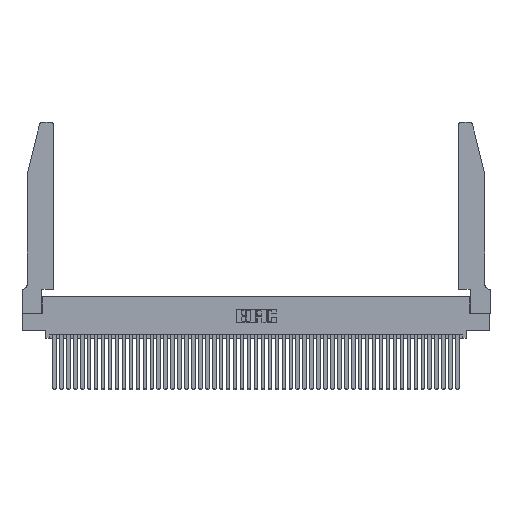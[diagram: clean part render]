
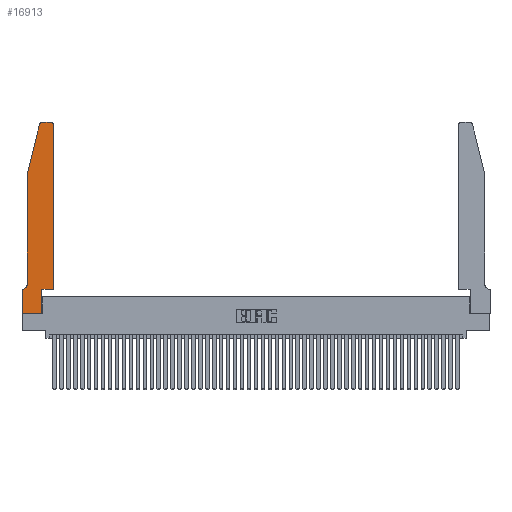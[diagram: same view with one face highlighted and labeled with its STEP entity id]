
A CAD part, top view. The second image highlights one B-rep face of the part: STEP entity #16913.
In plain terms, the highlighted planar face has unit normal (0, 0, 1).
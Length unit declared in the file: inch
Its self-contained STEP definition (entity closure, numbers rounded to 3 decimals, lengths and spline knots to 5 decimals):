
#142 = CARTESIAN_POINT ( 'NONE',  ( 0.25487, 2.72718, 0.37 ) ) ;
#521 = DIRECTION ( 'NONE',  ( 0., 1., 0. ) ) ;
#525 = LINE ( 'NONE', #27015, #20551 ) ;
#769 = VERTEX_POINT ( 'NONE', #40874 ) ;
#1063 = VECTOR ( 'NONE', #29589, 39.37008 ) ;
#1357 = ORIENTED_EDGE ( 'NONE', *, *, #36093, .T. ) ;
#1741 = EDGE_CURVE ( 'NONE', #16546, #47870, #20630, .T. ) ;
#1977 = DIRECTION ( 'NONE',  ( 0., 1., 0. ) ) ;
#2802 = EDGE_CURVE ( 'NONE', #31065, #769, #28888, .T. ) ;
#2891 = ORIENTED_EDGE ( 'NONE', *, *, #9325, .T. ) ;
#2956 = EDGE_CURVE ( 'NONE', #36001, #34604, #525, .T. ) ;
#3140 = VECTOR ( 'NONE', #14003, 39.37008 ) ;
#3671 = EDGE_CURVE ( 'NONE', #769, #18254, #16994, .T. ) ;
#3911 = EDGE_CURVE ( 'NONE', #32837, #31065, #13444, .T. ) ;
#4272 = DIRECTION ( 'NONE',  ( 1., 0., 0. ) ) ;
#4958 = DIRECTION ( 'NONE',  ( 1., 0., 0. ) ) ;
#6126 = DIRECTION ( 'NONE',  ( 0., 0., 1. ) ) ;
#7784 = VERTEX_POINT ( 'NONE', #32909 ) ;
#7906 = VECTOR ( 'NONE', #19432, 39.37008 ) ;
#8168 = CARTESIAN_POINT ( 'NONE',  ( 0.0755, 2., 0.37 ) ) ;
#8601 = EDGE_LOOP ( 'NONE', ( #1357, #22164, #12713, #36730, #45489, #14178, #24585, #2891, #27824, #33844, #46316, #10933 ) ) ;
#9325 = EDGE_CURVE ( 'NONE', #38260, #18668, #43754, .T. ) ;
#9332 = CARTESIAN_POINT ( 'NONE',  ( 0., 0.35, 0.37 ) ) ;
#9610 = CARTESIAN_POINT ( 'NONE',  ( 0., 0.35, 0.37 ) ) ;
#10315 = VERTEX_POINT ( 'NONE', #19049 ) ;
#10933 = ORIENTED_EDGE ( 'NONE', *, *, #25703, .T. ) ;
#12238 = VECTOR ( 'NONE', #23184, 39.37008 ) ;
#12713 = ORIENTED_EDGE ( 'NONE', *, *, #17390, .T. ) ;
#13444 = LINE ( 'NONE', #22144, #1063 ) ;
#14003 = DIRECTION ( 'NONE',  ( -1., 0., 0. ) ) ;
#14178 = ORIENTED_EDGE ( 'NONE', *, *, #3671, .T. ) ;
#14229 = CARTESIAN_POINT ( 'NONE',  ( 0.0755, 0.35, 0.37 ) ) ;
#14549 = CARTESIAN_POINT ( 'NONE',  ( 0.4205, 2.72, 0.37 ) ) ;
#14589 = VECTOR ( 'NONE', #1977, 39.37008 ) ;
#15662 = CARTESIAN_POINT ( 'NONE',  ( 0.0755, 2., 0.37 ) ) ;
#16546 = VERTEX_POINT ( 'NONE', #43193 ) ;
#16913 = ADVANCED_FACE ( 'NONE', ( #31694 ), #40052, .T. ) ;
#16994 = LINE ( 'NONE', #14229, #44630 ) ;
#17390 = EDGE_CURVE ( 'NONE', #47870, #32837, #26943, .T. ) ;
#17442 = EDGE_CURVE ( 'NONE', #18668, #10315, #37560, .T. ) ;
#17662 = DIRECTION ( 'NONE',  ( 1., 0., 0. ) ) ;
#17706 = DIRECTION ( 'NONE',  ( -1., 0., 0. ) ) ;
#18254 = VERTEX_POINT ( 'NONE', #9332 ) ;
#18338 = DIRECTION ( 'NONE',  ( 0., 0., -1. ) ) ;
#18668 = VERTEX_POINT ( 'NONE', #41861 ) ;
#19049 = CARTESIAN_POINT ( 'NONE',  ( 0.2865, 0.35, 0.37 ) ) ;
#19432 = DIRECTION ( 'NONE',  ( 0., -1., 0. ) ) ;
#19603 = CARTESIAN_POINT ( 'NONE',  ( 0., 0., 0.37 ) ) ;
#20551 = VECTOR ( 'NONE', #521, 39.37008 ) ;
#20630 = CIRCLE ( 'NONE', #36042, 0.03 ) ;
#22144 = CARTESIAN_POINT ( 'NONE',  ( 0.0755, 2., 0.37 ) ) ;
#22164 = ORIENTED_EDGE ( 'NONE', *, *, #1741, .T. ) ;
#22322 = CARTESIAN_POINT ( 'NONE',  ( 0., 0., 0.37 ) ) ;
#22633 = CARTESIAN_POINT ( 'NONE',  ( 0.4505, 2.72, 0.37 ) ) ;
#22659 = EDGE_CURVE ( 'NONE', #18254, #38260, #39142, .T. ) ;
#23184 = DIRECTION ( 'NONE',  ( -0.239, -0.971, 0. ) ) ;
#24585 = ORIENTED_EDGE ( 'NONE', *, *, #22659, .T. ) ;
#25005 = CARTESIAN_POINT ( 'NONE',  ( 0.4505, 0.35, 0.37 ) ) ;
#25560 = DIRECTION ( 'NONE',  ( 0., 0., 1. ) ) ;
#25703 = EDGE_CURVE ( 'NONE', #34604, #7784, #44085, .T. ) ;
#25897 = VECTOR ( 'NONE', #29331, 39.37008 ) ;
#26943 = LINE ( 'NONE', #15662, #12238 ) ;
#27015 = CARTESIAN_POINT ( 'NONE',  ( 0.4505, 0.35, 0.37 ) ) ;
#27170 = CARTESIAN_POINT ( 'NONE',  ( 0.284, 2.72, 0.37 ) ) ;
#27824 = ORIENTED_EDGE ( 'NONE', *, *, #17442, .T. ) ;
#28054 = AXIS2_PLACEMENT_3D ( 'NONE', #14549, #25560, #47782 ) ;
#28888 = CIRCLE ( 'NONE', #38283, 0.07 ) ;
#29331 = DIRECTION ( 'NONE',  ( 1., 0., 0. ) ) ;
#29589 = DIRECTION ( 'NONE',  ( 0., -1., 0. ) ) ;
#31065 = VERTEX_POINT ( 'NONE', #43310 ) ;
#31694 = FACE_OUTER_BOUND ( 'NONE', #8601, .T. ) ;
#32837 = VERTEX_POINT ( 'NONE', #8168 ) ;
#32909 = CARTESIAN_POINT ( 'NONE',  ( 0.4205, 2.75, 0.37 ) ) ;
#33058 = LINE ( 'NONE', #48221, #25897 ) ;
#33844 = ORIENTED_EDGE ( 'NONE', *, *, #42721, .T. ) ;
#34604 = VERTEX_POINT ( 'NONE', #22633 ) ;
#35227 = CARTESIAN_POINT ( 'NONE',  ( 0.2865, 0.35, 0.37 ) ) ;
#35390 = AXIS2_PLACEMENT_3D ( 'NONE', #9610, #6126, #17662 ) ;
#36001 = VERTEX_POINT ( 'NONE', #25005 ) ;
#36042 = AXIS2_PLACEMENT_3D ( 'NONE', #27170, #46253, #4958 ) ;
#36093 = EDGE_CURVE ( 'NONE', #7784, #16546, #37879, .T. ) ;
#36730 = ORIENTED_EDGE ( 'NONE', *, *, #3911, .T. ) ;
#37560 = LINE ( 'NONE', #35227, #14589 ) ;
#37879 = LINE ( 'NONE', #39880, #3140 ) ;
#38260 = VERTEX_POINT ( 'NONE', #22322 ) ;
#38283 = AXIS2_PLACEMENT_3D ( 'NONE', #48731, #18338, #44636 ) ;
#38497 = CARTESIAN_POINT ( 'NONE',  ( 0., 0., 0.37 ) ) ;
#38502 = VECTOR ( 'NONE', #4272, 39.37008 ) ;
#39142 = LINE ( 'NONE', #19603, #7906 ) ;
#39880 = CARTESIAN_POINT ( 'NONE',  ( 0.2605, 2.75, 0.37 ) ) ;
#40052 = PLANE ( 'NONE',  #35390 ) ;
#40874 = CARTESIAN_POINT ( 'NONE',  ( 0.0055, 0.35, 0.37 ) ) ;
#41861 = CARTESIAN_POINT ( 'NONE',  ( 0.2865, 0., 0.37 ) ) ;
#42721 = EDGE_CURVE ( 'NONE', #10315, #36001, #33058, .T. ) ;
#43193 = CARTESIAN_POINT ( 'NONE',  ( 0.284, 2.75, 0.37 ) ) ;
#43310 = CARTESIAN_POINT ( 'NONE',  ( 0.0755, 0.42, 0.37 ) ) ;
#43754 = LINE ( 'NONE', #38497, #38502 ) ;
#44085 = CIRCLE ( 'NONE', #28054, 0.03 ) ;
#44630 = VECTOR ( 'NONE', #17706, 39.37008 ) ;
#44636 = DIRECTION ( 'NONE',  ( -1., 0., 0. ) ) ;
#45489 = ORIENTED_EDGE ( 'NONE', *, *, #2802, .T. ) ;
#46253 = DIRECTION ( 'NONE',  ( 0., 0., 1. ) ) ;
#46316 = ORIENTED_EDGE ( 'NONE', *, *, #2956, .T. ) ;
#47782 = DIRECTION ( 'NONE',  ( 1., 0., 0. ) ) ;
#47870 = VERTEX_POINT ( 'NONE', #142 ) ;
#48221 = CARTESIAN_POINT ( 'NONE',  ( 0.4505, 0.35, 0.37 ) ) ;
#48731 = CARTESIAN_POINT ( 'NONE',  ( 0.0055, 0.42, 0.37 ) ) ;
